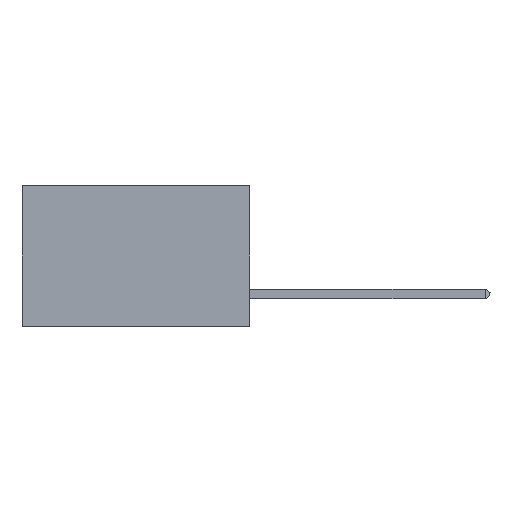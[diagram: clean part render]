
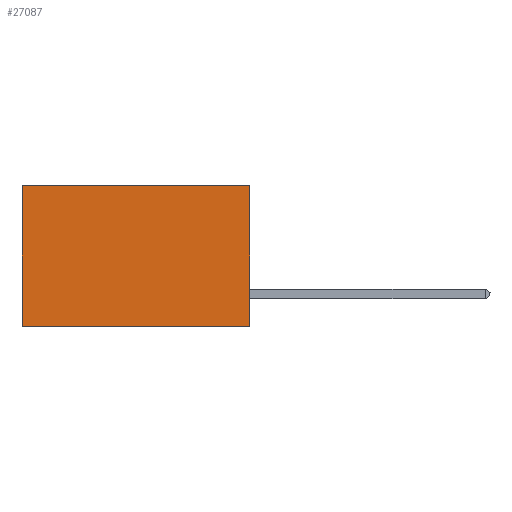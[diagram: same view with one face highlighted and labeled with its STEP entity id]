
A CAD part, left-side view. The second image highlights one B-rep face of the part: STEP entity #27087.
In plain terms, the highlighted planar face has unit normal (-1, 0, 0).
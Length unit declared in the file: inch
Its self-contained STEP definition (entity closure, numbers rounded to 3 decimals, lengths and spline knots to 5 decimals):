
#693 = ORIENTED_EDGE ( 'NONE', *, *, #37819, .F. ) ;
#852 = PLANE ( 'NONE',  #17713 ) ;
#3708 = DIRECTION ( 'NONE',  ( 0., 0., -1. ) ) ;
#6107 = CARTESIAN_POINT ( 'NONE',  ( 0.2875, 0., 0. ) ) ;
#9458 = VECTOR ( 'NONE', #25583, 39.37008 ) ;
#10103 = EDGE_CURVE ( 'NONE', #38033, #26579, #14488, .T. ) ;
#11193 = ORIENTED_EDGE ( 'NONE', *, *, #14750, .T. ) ;
#13148 = FACE_OUTER_BOUND ( 'NONE', #13740, .T. ) ;
#13254 = CARTESIAN_POINT ( 'NONE',  ( 0.2875, 0., 0. ) ) ;
#13740 = EDGE_LOOP ( 'NONE', ( #11193, #693, #21679, #36580 ) ) ;
#14276 = VECTOR ( 'NONE', #28629, 39.37008 ) ;
#14488 = LINE ( 'NONE', #13254, #9458 ) ;
#14750 = EDGE_CURVE ( 'NONE', #26579, #32749, #41697, .T. ) ;
#15825 = CARTESIAN_POINT ( 'NONE',  ( 0.2875, 0.6, -0.37 ) ) ;
#16274 = LINE ( 'NONE', #6107, #14276 ) ;
#16313 = EDGE_CURVE ( 'NONE', #38033, #25708, #16274, .T. ) ;
#17713 = AXIS2_PLACEMENT_3D ( 'NONE', #39222, #20054, #3708 ) ;
#20054 = DIRECTION ( 'NONE',  ( 1., 0., 0. ) ) ;
#21113 = CARTESIAN_POINT ( 'NONE',  ( 0.2875, 0., -0.37 ) ) ;
#21679 = ORIENTED_EDGE ( 'NONE', *, *, #16313, .F. ) ;
#22115 = VECTOR ( 'NONE', #35808, 39.37008 ) ;
#25583 = DIRECTION ( 'NONE',  ( 0., 1., 0. ) ) ;
#25708 = VERTEX_POINT ( 'NONE', #21113 ) ;
#26505 = VECTOR ( 'NONE', #39395, 39.37008 ) ;
#26579 = VERTEX_POINT ( 'NONE', #32490 ) ;
#27087 = ADVANCED_FACE ( 'NONE', ( #13148 ), #852, .F. ) ;
#28531 = CARTESIAN_POINT ( 'NONE',  ( 0.2875, 0.6, 0. ) ) ;
#28629 = DIRECTION ( 'NONE',  ( 0., 0., -1. ) ) ;
#31199 = CARTESIAN_POINT ( 'NONE',  ( 0.2875, 0., 0. ) ) ;
#32490 = CARTESIAN_POINT ( 'NONE',  ( 0.2875, 0.6, 0. ) ) ;
#32581 = CARTESIAN_POINT ( 'NONE',  ( 0.2875, 0., -0.37 ) ) ;
#32749 = VERTEX_POINT ( 'NONE', #15825 ) ;
#35808 = DIRECTION ( 'NONE',  ( 0., 1., 0. ) ) ;
#36580 = ORIENTED_EDGE ( 'NONE', *, *, #10103, .T. ) ;
#37819 = EDGE_CURVE ( 'NONE', #25708, #32749, #40848, .T. ) ;
#38033 = VERTEX_POINT ( 'NONE', #31199 ) ;
#39222 = CARTESIAN_POINT ( 'NONE',  ( 0.2875, 0., 0. ) ) ;
#39395 = DIRECTION ( 'NONE',  ( 0., 0., -1. ) ) ;
#40848 = LINE ( 'NONE', #32581, #22115 ) ;
#41697 = LINE ( 'NONE', #28531, #26505 ) ;
